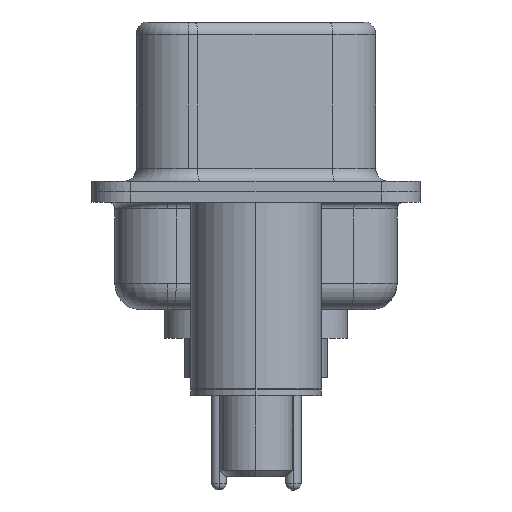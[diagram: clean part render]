
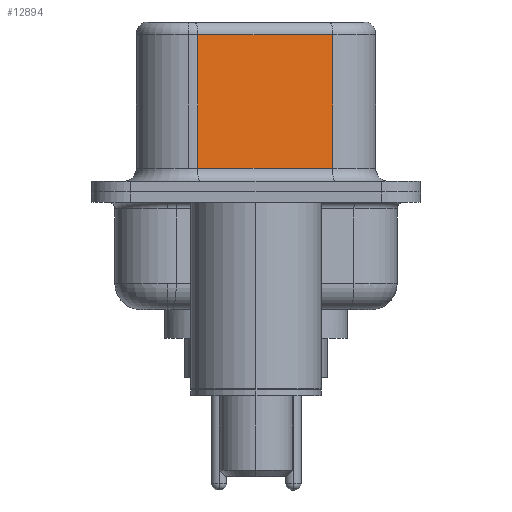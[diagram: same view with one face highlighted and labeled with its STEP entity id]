
A CAD part, left-side view. The second image highlights one B-rep face of the part: STEP entity #12894.
In plain terms, the highlighted planar face has unit normal (-0.985, -0.174, 0).
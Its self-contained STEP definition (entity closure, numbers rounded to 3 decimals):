
#301 = AXIS2_PLACEMENT_3D ( 'NONE', #12909, #5696, #15822 ) ;
#783 = CARTESIAN_POINT ( 'NONE',  ( 3.675, 2.233, 6.02 ) ) ;
#797 = LINE ( 'NONE', #5800, #16366 ) ;
#811 = DIRECTION ( 'NONE',  ( -0.174, 0.985, 0. ) ) ;
#892 = CARTESIAN_POINT ( 'NONE',  ( 4.585, -2.927, 6.02 ) ) ;
#2264 = CARTESIAN_POINT ( 'NONE',  ( 4.585, -2.927, 0.9 ) ) ;
#3090 = ORIENTED_EDGE ( 'NONE', *, *, #5709, .T. ) ;
#3827 = ORIENTED_EDGE ( 'NONE', *, *, #7698, .F. ) ;
#4186 = PLANE ( 'NONE',  #301 ) ;
#5476 = ORIENTED_EDGE ( 'NONE', *, *, #9426, .T. ) ;
#5567 = VERTEX_POINT ( 'NONE', #2264 ) ;
#5696 = DIRECTION ( 'NONE',  ( 0.985, 0.174, 0. ) ) ;
#5709 = EDGE_CURVE ( 'NONE', #10327, #5567, #8476, .T. ) ;
#5800 = CARTESIAN_POINT ( 'NONE',  ( 3.675, 2.233, 6.52 ) ) ;
#6696 = DIRECTION ( 'NONE',  ( 0., 0., -1. ) ) ;
#6737 = CARTESIAN_POINT ( 'NONE',  ( 4.585, -2.927, 6.52 ) ) ;
#7275 = VECTOR ( 'NONE', #6696, 1000. ) ;
#7698 = EDGE_CURVE ( 'NONE', #13880, #5567, #18754, .T. ) ;
#8476 = LINE ( 'NONE', #11255, #12264 ) ;
#9272 = EDGE_LOOP ( 'NONE', ( #3827, #5476, #16557, #3090 ) ) ;
#9301 = DIRECTION ( 'NONE',  ( 0.174, -0.985, 0. ) ) ;
#9426 = EDGE_CURVE ( 'NONE', #13880, #15988, #15998, .T. ) ;
#9991 = CARTESIAN_POINT ( 'NONE',  ( 4.585, -2.927, 6.02 ) ) ;
#10327 = VERTEX_POINT ( 'NONE', #12969 ) ;
#11255 = CARTESIAN_POINT ( 'NONE',  ( 4.585, -2.927, 0.9 ) ) ;
#11681 = VECTOR ( 'NONE', #811, 1000. ) ;
#12264 = VECTOR ( 'NONE', #9301, 1000. ) ;
#12894 = ADVANCED_FACE ( 'NONE', ( #17976 ), #4186, .F. ) ;
#12909 = CARTESIAN_POINT ( 'NONE',  ( 4.585, -2.927, 6.52 ) ) ;
#12969 = CARTESIAN_POINT ( 'NONE',  ( 3.675, 2.233, 0.9 ) ) ;
#13880 = VERTEX_POINT ( 'NONE', #9991 ) ;
#13941 = EDGE_CURVE ( 'NONE', #15988, #10327, #797, .T. ) ;
#15822 = DIRECTION ( 'NONE',  ( -0.174, 0.985, 0. ) ) ;
#15988 = VERTEX_POINT ( 'NONE', #783 ) ;
#15998 = LINE ( 'NONE', #892, #11681 ) ;
#16366 = VECTOR ( 'NONE', #17352, 1000. ) ;
#16557 = ORIENTED_EDGE ( 'NONE', *, *, #13941, .T. ) ;
#17352 = DIRECTION ( 'NONE',  ( 0., 0., -1. ) ) ;
#17976 = FACE_OUTER_BOUND ( 'NONE', #9272, .T. ) ;
#18754 = LINE ( 'NONE', #6737, #7275 ) ;
